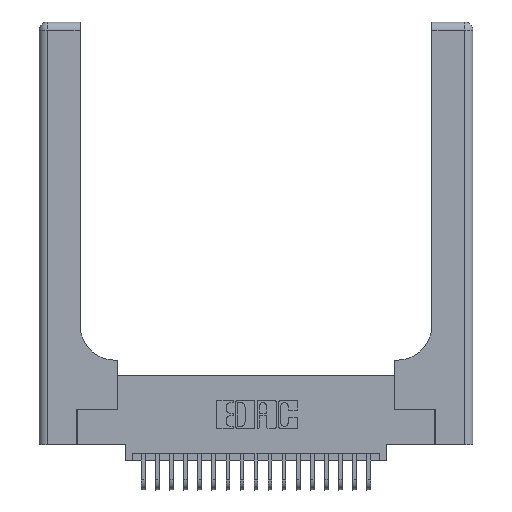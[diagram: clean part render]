
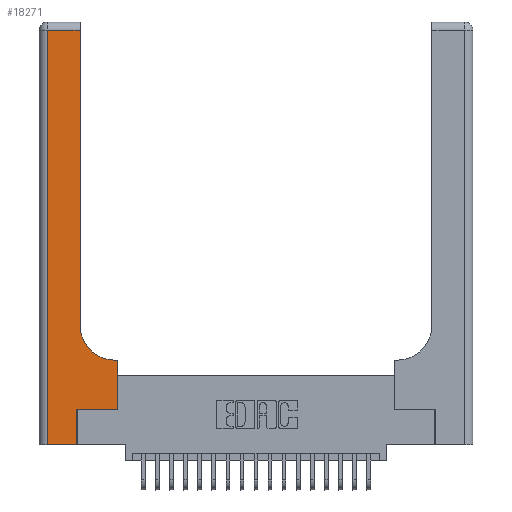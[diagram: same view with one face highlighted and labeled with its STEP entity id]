
A CAD part, top view. The second image highlights one B-rep face of the part: STEP entity #18271.
In plain terms, the highlighted planar face has unit normal (0, 0, 1).
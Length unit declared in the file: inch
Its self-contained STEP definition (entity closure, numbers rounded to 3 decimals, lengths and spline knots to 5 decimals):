
#510 = EDGE_CURVE ( 'NONE', #7905, #14159, #2530, .T. ) ;
#735 = CARTESIAN_POINT ( 'NONE',  ( 0.5585, 0.6, 0.37 ) ) ;
#1283 = VECTOR ( 'NONE', #20944, 39.37008 ) ;
#1726 = EDGE_CURVE ( 'NONE', #8854, #10781, #13596, .T. ) ;
#1908 = VECTOR ( 'NONE', #19108, 39.37008 ) ;
#1995 = CARTESIAN_POINT ( 'NONE',  ( 0.269, 0., 0.37 ) ) ;
#2010 = VECTOR ( 'NONE', #22558, 39.37008 ) ;
#2372 = DIRECTION ( 'NONE',  ( 0., 0., -1. ) ) ;
#2530 = CIRCLE ( 'NONE', #2732, 0.25 ) ;
#2562 = PLANE ( 'NONE',  #10770 ) ;
#2683 = DIRECTION ( 'NONE',  ( 1., 0., 0. ) ) ;
#2721 = EDGE_CURVE ( 'NONE', #7691, #14227, #21620, .T. ) ;
#2732 = AXIS2_PLACEMENT_3D ( 'NONE', #15285, #2372, #6199 ) ;
#3127 = DIRECTION ( 'NONE',  ( 0., 1., 0. ) ) ;
#3171 = LINE ( 'NONE', #4308, #2010 ) ;
#4277 = CARTESIAN_POINT ( 'NONE',  ( 0.5585, 0.25, 0.37 ) ) ;
#4308 = CARTESIAN_POINT ( 'NONE',  ( 0.269, 0.25, 0.37 ) ) ;
#5163 = LINE ( 'NONE', #7867, #12010 ) ;
#5562 = CARTESIAN_POINT ( 'NONE',  ( 0.06, 0., 0.37 ) ) ;
#5683 = LINE ( 'NONE', #13477, #19448 ) ;
#6174 = EDGE_CURVE ( 'NONE', #21303, #15294, #5683, .T. ) ;
#6199 = DIRECTION ( 'NONE',  ( 1., 0., 0. ) ) ;
#6386 = CARTESIAN_POINT ( 'NONE',  ( 0., 2.94, 0.37 ) ) ;
#6400 = VECTOR ( 'NONE', #3127, 39.37008 ) ;
#7546 = ORIENTED_EDGE ( 'NONE', *, *, #10406, .T. ) ;
#7691 = VERTEX_POINT ( 'NONE', #15622 ) ;
#7822 = DIRECTION ( 'NONE',  ( 0., 0., -1. ) ) ;
#7867 = CARTESIAN_POINT ( 'NONE',  ( 0., 0., 0.37 ) ) ;
#7905 = VERTEX_POINT ( 'NONE', #23287 ) ;
#8133 = CARTESIAN_POINT ( 'NONE',  ( 0.2915, 0.6, 0.37 ) ) ;
#8854 = VERTEX_POINT ( 'NONE', #1995 ) ;
#9032 = EDGE_CURVE ( 'NONE', #10075, #21303, #17578, .T. ) ;
#9800 = CARTESIAN_POINT ( 'NONE',  ( 0.269, 0.25, 0.37 ) ) ;
#9980 = DIRECTION ( 'NONE',  ( 0., -1., 0. ) ) ;
#10075 = VERTEX_POINT ( 'NONE', #16703 ) ;
#10152 = CARTESIAN_POINT ( 'NONE',  ( 0.269, 0., 0.37 ) ) ;
#10406 = EDGE_CURVE ( 'NONE', #14159, #10075, #17260, .T. ) ;
#10770 = AXIS2_PLACEMENT_3D ( 'NONE', #22480, #7822, #22640 ) ;
#10781 = VERTEX_POINT ( 'NONE', #9800 ) ;
#10799 = ORIENTED_EDGE ( 'NONE', *, *, #12120, .T. ) ;
#12010 = VECTOR ( 'NONE', #2683, 39.37008 ) ;
#12120 = EDGE_CURVE ( 'NONE', #15294, #8854, #5163, .T. ) ;
#12732 = VECTOR ( 'NONE', #17055, 39.37008 ) ;
#13477 = CARTESIAN_POINT ( 'NONE',  ( 0.06, 3., 0.37 ) ) ;
#13596 = LINE ( 'NONE', #10152, #1908 ) ;
#13718 = ORIENTED_EDGE ( 'NONE', *, *, #510, .T. ) ;
#14159 = VERTEX_POINT ( 'NONE', #18486 ) ;
#14227 = VERTEX_POINT ( 'NONE', #735 ) ;
#14910 = EDGE_CURVE ( 'NONE', #10781, #7691, #3171, .T. ) ;
#15285 = CARTESIAN_POINT ( 'NONE',  ( 0.5415, 0.85, 0.37 ) ) ;
#15294 = VERTEX_POINT ( 'NONE', #5562 ) ;
#15622 = CARTESIAN_POINT ( 'NONE',  ( 0.5585, 0.25, 0.37 ) ) ;
#16703 = CARTESIAN_POINT ( 'NONE',  ( 0.2915, 2.94, 0.37 ) ) ;
#16742 = EDGE_CURVE ( 'NONE', #14227, #7905, #22259, .T. ) ;
#17055 = DIRECTION ( 'NONE',  ( 0., 1., 0. ) ) ;
#17260 = LINE ( 'NONE', #23374, #6400 ) ;
#17578 = LINE ( 'NONE', #6386, #1283 ) ;
#17841 = ORIENTED_EDGE ( 'NONE', *, *, #16742, .T. ) ;
#18271 = ADVANCED_FACE ( 'NONE', ( #21639 ), #2562, .F. ) ;
#18486 = CARTESIAN_POINT ( 'NONE',  ( 0.2915, 0.85, 0.37 ) ) ;
#18905 = ORIENTED_EDGE ( 'NONE', *, *, #6174, .T. ) ;
#19100 = DIRECTION ( 'NONE',  ( -1., 0., 0. ) ) ;
#19108 = DIRECTION ( 'NONE',  ( 0., 1., 0. ) ) ;
#19448 = VECTOR ( 'NONE', #9980, 39.37008 ) ;
#20135 = ORIENTED_EDGE ( 'NONE', *, *, #1726, .T. ) ;
#20944 = DIRECTION ( 'NONE',  ( -1., 0., 0. ) ) ;
#21303 = VERTEX_POINT ( 'NONE', #22885 ) ;
#21620 = LINE ( 'NONE', #4277, #12732 ) ;
#21639 = FACE_OUTER_BOUND ( 'NONE', #22257, .T. ) ;
#21679 = ORIENTED_EDGE ( 'NONE', *, *, #14910, .T. ) ;
#21688 = VECTOR ( 'NONE', #19100, 39.37008 ) ;
#21860 = ORIENTED_EDGE ( 'NONE', *, *, #9032, .T. ) ;
#22257 = EDGE_LOOP ( 'NONE', ( #7546, #21860, #18905, #10799, #20135, #21679, #22564, #17841, #13718 ) ) ;
#22259 = LINE ( 'NONE', #8133, #21688 ) ;
#22480 = CARTESIAN_POINT ( 'NONE',  ( 0., 3., 0.37 ) ) ;
#22558 = DIRECTION ( 'NONE',  ( 1., 0., 0. ) ) ;
#22564 = ORIENTED_EDGE ( 'NONE', *, *, #2721, .T. ) ;
#22640 = DIRECTION ( 'NONE',  ( -1., 0., 0. ) ) ;
#22885 = CARTESIAN_POINT ( 'NONE',  ( 0.06, 2.94, 0.37 ) ) ;
#23287 = CARTESIAN_POINT ( 'NONE',  ( 0.5415, 0.6, 0.37 ) ) ;
#23374 = CARTESIAN_POINT ( 'NONE',  ( 0.2915, 3., 0.37 ) ) ;
